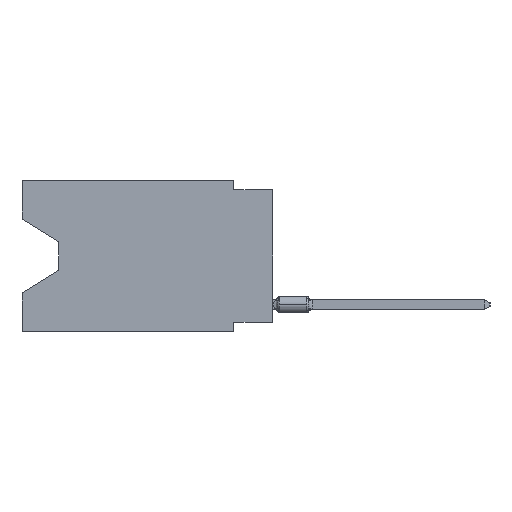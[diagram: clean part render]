
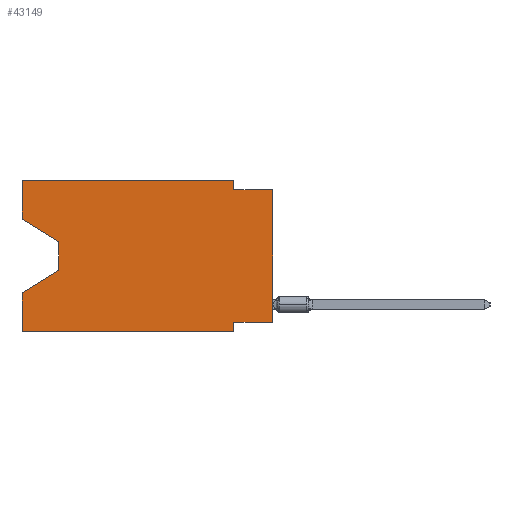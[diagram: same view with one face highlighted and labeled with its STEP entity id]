
A CAD part, left-side view. The second image highlights one B-rep face of the part: STEP entity #43149.
In plain terms, the highlighted planar face has unit normal (-1, 0, 0).
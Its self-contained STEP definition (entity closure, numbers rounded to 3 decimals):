
#184 = VECTOR ( 'NONE', #7859, 1000. ) ;
#1327 = CARTESIAN_POINT ( 'NONE',  ( 0., 16.383, -2.546 ) ) ;
#2058 = DIRECTION ( 'NONE',  ( 0., 0., 1. ) ) ;
#2348 = CARTESIAN_POINT ( 'NONE',  ( 0., 2.54, -9.906 ) ) ;
#2496 = DIRECTION ( 'NONE',  ( 0., 0., -1. ) ) ;
#2530 = DIRECTION ( 'NONE',  ( 0., -0.855, -0.519 ) ) ;
#3670 = CARTESIAN_POINT ( 'NONE',  ( 0., 16.383, 0. ) ) ;
#4360 = LINE ( 'NONE', #34376, #7478 ) ;
#5065 = VERTEX_POINT ( 'NONE', #38495 ) ;
#5417 = CARTESIAN_POINT ( 'NONE',  ( 0., 13.97, -4.013 ) ) ;
#6206 = VECTOR ( 'NONE', #2058, 1000. ) ;
#6590 = DIRECTION ( 'NONE',  ( 1., 0., 0. ) ) ;
#6619 = CARTESIAN_POINT ( 'NONE',  ( 0., 2.54, 0. ) ) ;
#7261 = DIRECTION ( 'NONE',  ( 0., 0., -1. ) ) ;
#7478 = VECTOR ( 'NONE', #13968, 1000. ) ;
#7556 = VERTEX_POINT ( 'NONE', #1327 ) ;
#7859 = DIRECTION ( 'NONE',  ( 0., 0.855, -0.519 ) ) ;
#9249 = ORIENTED_EDGE ( 'NONE', *, *, #23013, .T. ) ;
#9314 = VERTEX_POINT ( 'NONE', #39151 ) ;
#9448 = EDGE_CURVE ( 'NONE', #36473, #20208, #18542, .T. ) ;
#9906 = EDGE_CURVE ( 'NONE', #40028, #33681, #16451, .T. ) ;
#10487 = CARTESIAN_POINT ( 'NONE',  ( 0., 16.383, -9.906 ) ) ;
#10611 = CARTESIAN_POINT ( 'NONE',  ( 0., 16.383, -7.36 ) ) ;
#10796 = VECTOR ( 'NONE', #2496, 1000. ) ;
#11396 = ORIENTED_EDGE ( 'NONE', *, *, #36350, .T. ) ;
#12006 = CARTESIAN_POINT ( 'NONE',  ( 0., 13.97, -5.893 ) ) ;
#12269 = DIRECTION ( 'NONE',  ( 0., 0., 1. ) ) ;
#13312 = LINE ( 'NONE', #30136, #32167 ) ;
#13444 = ORIENTED_EDGE ( 'NONE', *, *, #37127, .T. ) ;
#13508 = PLANE ( 'NONE',  #37460 ) ;
#13968 = DIRECTION ( 'NONE',  ( 0., -1., 0. ) ) ;
#13971 = VERTEX_POINT ( 'NONE', #10611 ) ;
#14137 = ORIENTED_EDGE ( 'NONE', *, *, #9448, .F. ) ;
#15086 = EDGE_CURVE ( 'NONE', #29319, #13971, #21877, .T. ) ;
#15183 = CARTESIAN_POINT ( 'NONE',  ( 0., 16.383, 0. ) ) ;
#15397 = VERTEX_POINT ( 'NONE', #20499 ) ;
#15811 = DIRECTION ( 'NONE',  ( 0., 0., -1. ) ) ;
#16288 = EDGE_CURVE ( 'NONE', #18790, #13971, #21712, .T. ) ;
#16451 = LINE ( 'NONE', #2348, #34043 ) ;
#16684 = CARTESIAN_POINT ( 'NONE',  ( 0., 0., -9.271 ) ) ;
#17139 = ORIENTED_EDGE ( 'NONE', *, *, #34107, .F. ) ;
#17516 = EDGE_LOOP ( 'NONE', ( #9249, #31524, #29404, #34551, #13444, #42197, #17571, #11396, #17139, #19333, #14137, #36050 ) ) ;
#17571 = ORIENTED_EDGE ( 'NONE', *, *, #19062, .F. ) ;
#17641 = VECTOR ( 'NONE', #12269, 1000. ) ;
#18398 = VECTOR ( 'NONE', #37596, 1000. ) ;
#18542 = LINE ( 'NONE', #15183, #28288 ) ;
#18597 = DIRECTION ( 'NONE',  ( 0., 0., 1. ) ) ;
#18790 = VERTEX_POINT ( 'NONE', #12006 ) ;
#19062 = EDGE_CURVE ( 'NONE', #9314, #40028, #40876, .T. ) ;
#19333 = ORIENTED_EDGE ( 'NONE', *, *, #22330, .F. ) ;
#20176 = CARTESIAN_POINT ( 'NONE',  ( 0., 16.383, -9.906 ) ) ;
#20197 = LINE ( 'NONE', #33206, #34789 ) ;
#20208 = VERTEX_POINT ( 'NONE', #6619 ) ;
#20499 = CARTESIAN_POINT ( 'NONE',  ( 0., 0., -0.635 ) ) ;
#21712 = LINE ( 'NONE', #28888, #184 ) ;
#21877 = LINE ( 'NONE', #25454, #17641 ) ;
#21936 = CARTESIAN_POINT ( 'NONE',  ( 0., 16.383, 0. ) ) ;
#22330 = EDGE_CURVE ( 'NONE', #20208, #5065, #13312, .T. ) ;
#22471 = CARTESIAN_POINT ( 'NONE',  ( 0., 2.54, -9.906 ) ) ;
#22634 = LINE ( 'NONE', #5417, #10796 ) ;
#23013 = EDGE_CURVE ( 'NONE', #7556, #33463, #20197, .T. ) ;
#23904 = LINE ( 'NONE', #10487, #18398 ) ;
#24052 = CARTESIAN_POINT ( 'NONE',  ( 0., 13.97, -4.013 ) ) ;
#24477 = FACE_OUTER_BOUND ( 'NONE', #17516, .T. ) ;
#25454 = CARTESIAN_POINT ( 'NONE',  ( 0., 16.383, 0. ) ) ;
#26301 = DIRECTION ( 'NONE',  ( 0., 0., -1. ) ) ;
#28288 = VECTOR ( 'NONE', #28838, 1000. ) ;
#28838 = DIRECTION ( 'NONE',  ( 0., -1., 0. ) ) ;
#28888 = CARTESIAN_POINT ( 'NONE',  ( 0., 13.97, -5.893 ) ) ;
#28947 = CARTESIAN_POINT ( 'NONE',  ( 0., 0., 0. ) ) ;
#29319 = VERTEX_POINT ( 'NONE', #20176 ) ;
#29404 = ORIENTED_EDGE ( 'NONE', *, *, #16288, .T. ) ;
#29824 = EDGE_CURVE ( 'NONE', #33463, #18790, #22634, .T. ) ;
#30136 = CARTESIAN_POINT ( 'NONE',  ( 0., 2.54, 0. ) ) ;
#31524 = ORIENTED_EDGE ( 'NONE', *, *, #29824, .T. ) ;
#32167 = VECTOR ( 'NONE', #15811, 1000. ) ;
#33206 = CARTESIAN_POINT ( 'NONE',  ( 0., 16.383, -2.546 ) ) ;
#33463 = VERTEX_POINT ( 'NONE', #24052 ) ;
#33681 = VERTEX_POINT ( 'NONE', #22471 ) ;
#34043 = VECTOR ( 'NONE', #26301, 1000. ) ;
#34107 = EDGE_CURVE ( 'NONE', #5065, #15397, #4360, .T. ) ;
#34376 = CARTESIAN_POINT ( 'NONE',  ( 0., 0., -0.635 ) ) ;
#34551 = ORIENTED_EDGE ( 'NONE', *, *, #15086, .F. ) ;
#34789 = VECTOR ( 'NONE', #2530, 1000. ) ;
#36050 = ORIENTED_EDGE ( 'NONE', *, *, #36816, .F. ) ;
#36350 = EDGE_CURVE ( 'NONE', #9314, #15397, #38817, .T. ) ;
#36473 = VERTEX_POINT ( 'NONE', #39693 ) ;
#36816 = EDGE_CURVE ( 'NONE', #7556, #36473, #38975, .T. ) ;
#37127 = EDGE_CURVE ( 'NONE', #29319, #33681, #23904, .T. ) ;
#37460 = AXIS2_PLACEMENT_3D ( 'NONE', #3670, #6590, #7261 ) ;
#37504 = DIRECTION ( 'NONE',  ( 0., 1., 0. ) ) ;
#37596 = DIRECTION ( 'NONE',  ( 0., -1., 0. ) ) ;
#38126 = CARTESIAN_POINT ( 'NONE',  ( 0., 2.54, -9.271 ) ) ;
#38495 = CARTESIAN_POINT ( 'NONE',  ( 0., 2.54, -0.635 ) ) ;
#38817 = LINE ( 'NONE', #28947, #6206 ) ;
#38975 = LINE ( 'NONE', #21936, #43451 ) ;
#39151 = CARTESIAN_POINT ( 'NONE',  ( 0., 0., -9.271 ) ) ;
#39693 = CARTESIAN_POINT ( 'NONE',  ( 0., 16.383, 0. ) ) ;
#40028 = VERTEX_POINT ( 'NONE', #38126 ) ;
#40876 = LINE ( 'NONE', #16684, #43534 ) ;
#42197 = ORIENTED_EDGE ( 'NONE', *, *, #9906, .F. ) ;
#43149 = ADVANCED_FACE ( 'NONE', ( #24477 ), #13508, .F. ) ;
#43451 = VECTOR ( 'NONE', #18597, 1000. ) ;
#43534 = VECTOR ( 'NONE', #37504, 1000. ) ;
